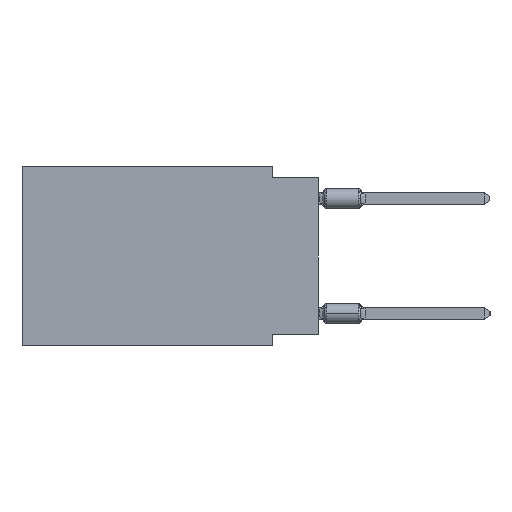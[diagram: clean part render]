
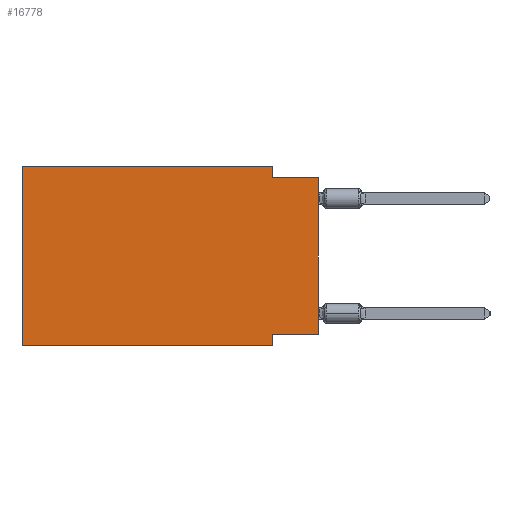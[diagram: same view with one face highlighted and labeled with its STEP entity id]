
A CAD part, left-side view. The second image highlights one B-rep face of the part: STEP entity #16778.
In plain terms, the highlighted planar face has unit normal (-1, 0, 0).
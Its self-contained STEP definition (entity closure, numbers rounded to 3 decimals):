
#1060 = EDGE_CURVE ( 'NONE', #56056, #54991, #4498, .T. ) ;
#2117 = VERTEX_POINT ( 'NONE', #40403 ) ;
#2419 = ORIENTED_EDGE ( 'NONE', *, *, #35748, .F. ) ;
#3006 = LINE ( 'NONE', #31870, #28379 ) ;
#4498 = LINE ( 'NONE', #55289, #13807 ) ;
#4941 = VECTOR ( 'NONE', #52882, 1000. ) ;
#5034 = CARTESIAN_POINT ( 'NONE',  ( 0., 16.383, 0. ) ) ;
#7722 = CARTESIAN_POINT ( 'NONE',  ( 0., 2.54, 0. ) ) ;
#9231 = ORIENTED_EDGE ( 'NONE', *, *, #1060, .F. ) ;
#9418 = CARTESIAN_POINT ( 'NONE',  ( 0., 16.383, 0. ) ) ;
#12950 = AXIS2_PLACEMENT_3D ( 'NONE', #17329, #22227, #36960 ) ;
#13807 = VECTOR ( 'NONE', #64169, 1000. ) ;
#14904 = VERTEX_POINT ( 'NONE', #55084 ) ;
#14949 = EDGE_CURVE ( 'NONE', #31828, #2117, #50824, .T. ) ;
#16114 = VECTOR ( 'NONE', #53627, 1000. ) ;
#16413 = CARTESIAN_POINT ( 'NONE',  ( 0., 0., 0. ) ) ;
#16778 = ADVANCED_FACE ( 'NONE', ( #48110 ), #32044, .F. ) ;
#17329 = CARTESIAN_POINT ( 'NONE',  ( 0., 16.383, 0. ) ) ;
#17920 = CARTESIAN_POINT ( 'NONE',  ( 0., 2.54, -9.906 ) ) ;
#20003 = CARTESIAN_POINT ( 'NONE',  ( 0., 16.383, -9.906 ) ) ;
#21414 = ORIENTED_EDGE ( 'NONE', *, *, #28638, .F. ) ;
#22227 = DIRECTION ( 'NONE',  ( 1., 0., 0. ) ) ;
#25740 = CARTESIAN_POINT ( 'NONE',  ( 0., 16.383, -9.906 ) ) ;
#25815 = VERTEX_POINT ( 'NONE', #20003 ) ;
#28379 = VECTOR ( 'NONE', #51884, 1000. ) ;
#28638 = EDGE_CURVE ( 'NONE', #31828, #14904, #3006, .T. ) ;
#29612 = EDGE_CURVE ( 'NONE', #14904, #40570, #38536, .T. ) ;
#31301 = VECTOR ( 'NONE', #50320, 1000. ) ;
#31828 = VERTEX_POINT ( 'NONE', #34112 ) ;
#31870 = CARTESIAN_POINT ( 'NONE',  ( 0., 0., -9.271 ) ) ;
#32044 = PLANE ( 'NONE',  #12950 ) ;
#32130 = VECTOR ( 'NONE', #45027, 1000. ) ;
#32510 = ORIENTED_EDGE ( 'NONE', *, *, #14949, .T. ) ;
#33175 = CARTESIAN_POINT ( 'NONE',  ( 0., 0., -0.635 ) ) ;
#34112 = CARTESIAN_POINT ( 'NONE',  ( 0., 0., -9.271 ) ) ;
#35748 = EDGE_CURVE ( 'NONE', #54991, #60912, #43782, .T. ) ;
#36960 = DIRECTION ( 'NONE',  ( 0., 0., -1. ) ) ;
#37320 = ORIENTED_EDGE ( 'NONE', *, *, #29612, .F. ) ;
#38536 = LINE ( 'NONE', #17920, #59883 ) ;
#39172 = DIRECTION ( 'NONE',  ( 0., 0., -1. ) ) ;
#40372 = EDGE_CURVE ( 'NONE', #25815, #40570, #64752, .T. ) ;
#40403 = CARTESIAN_POINT ( 'NONE',  ( 0., 0., -0.635 ) ) ;
#40570 = VERTEX_POINT ( 'NONE', #58764 ) ;
#40744 = LINE ( 'NONE', #5034, #32130 ) ;
#42581 = ORIENTED_EDGE ( 'NONE', *, *, #49392, .F. ) ;
#43782 = LINE ( 'NONE', #60719, #16114 ) ;
#45027 = DIRECTION ( 'NONE',  ( 0., 0., 1. ) ) ;
#48110 = FACE_OUTER_BOUND ( 'NONE', #62729, .T. ) ;
#49212 = EDGE_CURVE ( 'NONE', #25815, #56056, #40744, .T. ) ;
#49392 = EDGE_CURVE ( 'NONE', #60912, #2117, #63348, .T. ) ;
#49978 = ORIENTED_EDGE ( 'NONE', *, *, #40372, .T. ) ;
#50320 = DIRECTION ( 'NONE',  ( 0., -1., 0. ) ) ;
#50824 = LINE ( 'NONE', #16413, #59936 ) ;
#51884 = DIRECTION ( 'NONE',  ( 0., 1., 0. ) ) ;
#52882 = DIRECTION ( 'NONE',  ( 0., -1., 0. ) ) ;
#53627 = DIRECTION ( 'NONE',  ( 0., 0., -1. ) ) ;
#53739 = ORIENTED_EDGE ( 'NONE', *, *, #49212, .F. ) ;
#54991 = VERTEX_POINT ( 'NONE', #7722 ) ;
#55084 = CARTESIAN_POINT ( 'NONE',  ( 0., 2.54, -9.271 ) ) ;
#55289 = CARTESIAN_POINT ( 'NONE',  ( 0., 16.383, 0. ) ) ;
#56056 = VERTEX_POINT ( 'NONE', #9418 ) ;
#58764 = CARTESIAN_POINT ( 'NONE',  ( 0., 2.54, -9.906 ) ) ;
#59883 = VECTOR ( 'NONE', #39172, 1000. ) ;
#59936 = VECTOR ( 'NONE', #60658, 1000. ) ;
#60658 = DIRECTION ( 'NONE',  ( 0., 0., 1. ) ) ;
#60719 = CARTESIAN_POINT ( 'NONE',  ( 0., 2.54, 0. ) ) ;
#60912 = VERTEX_POINT ( 'NONE', #62676 ) ;
#62676 = CARTESIAN_POINT ( 'NONE',  ( 0., 2.54, -0.635 ) ) ;
#62729 = EDGE_LOOP ( 'NONE', ( #32510, #42581, #2419, #9231, #53739, #49978, #37320, #21414 ) ) ;
#63348 = LINE ( 'NONE', #33175, #4941 ) ;
#64169 = DIRECTION ( 'NONE',  ( 0., -1., 0. ) ) ;
#64752 = LINE ( 'NONE', #25740, #31301 ) ;
